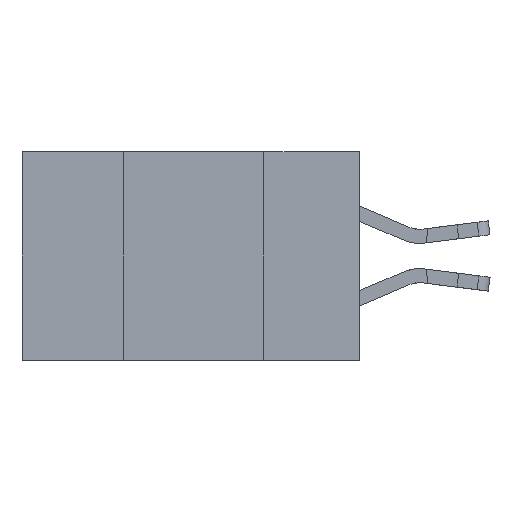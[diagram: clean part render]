
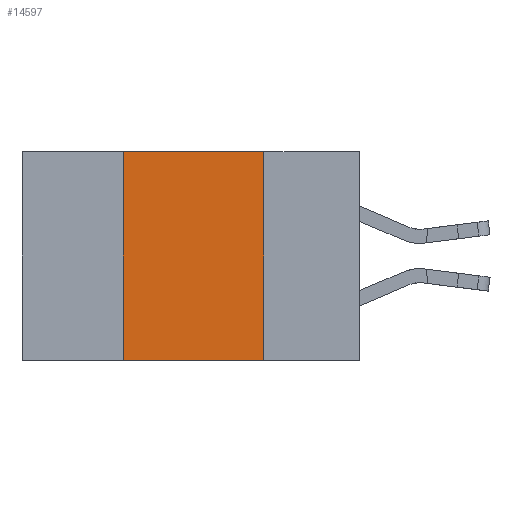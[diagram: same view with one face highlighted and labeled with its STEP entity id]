
A CAD part, left-side view. The second image highlights one B-rep face of the part: STEP entity #14597.
In plain terms, the highlighted planar face has unit normal (-1, 0, 0).
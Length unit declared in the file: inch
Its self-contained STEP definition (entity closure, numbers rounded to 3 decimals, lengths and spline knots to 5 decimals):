
#105 = FACE_OUTER_BOUND ( 'NONE', #21071, .T. ) ;
#202 = ORIENTED_EDGE ( 'NONE', *, *, #13890, .T. ) ;
#730 = DIRECTION ( 'NONE',  ( 0., 0., 1. ) ) ;
#1035 = CARTESIAN_POINT ( 'NONE',  ( 0., 0.42, -0.37 ) ) ;
#1326 = DIRECTION ( 'NONE',  ( 1., 0., 0. ) ) ;
#1566 = DIRECTION ( 'NONE',  ( 0., -1., 0. ) ) ;
#2985 = DIRECTION ( 'NONE',  ( 0., 0., -1. ) ) ;
#4285 = CARTESIAN_POINT ( 'NONE',  ( 0., 0.6, 0. ) ) ;
#6379 = VECTOR ( 'NONE', #1566, 39.37008 ) ;
#7774 = EDGE_CURVE ( 'NONE', #9730, #18237, #19618, .T. ) ;
#7858 = ORIENTED_EDGE ( 'NONE', *, *, #7774, .F. ) ;
#8973 = CARTESIAN_POINT ( 'NONE',  ( 0., 0.17, -0.37 ) ) ;
#9730 = VERTEX_POINT ( 'NONE', #22725 ) ;
#10866 = ORIENTED_EDGE ( 'NONE', *, *, #15050, .F. ) ;
#11631 = VERTEX_POINT ( 'NONE', #8973 ) ;
#12085 = CARTESIAN_POINT ( 'NONE',  ( 0., 0.6, 0. ) ) ;
#13846 = DIRECTION ( 'NONE',  ( 0., 0., -1. ) ) ;
#13890 = EDGE_CURVE ( 'NONE', #20618, #11631, #20948, .T. ) ;
#14597 = ADVANCED_FACE ( 'NONE', ( #105 ), #22437, .F. ) ;
#15050 = EDGE_CURVE ( 'NONE', #20618, #9730, #18485, .T. ) ;
#15930 = AXIS2_PLACEMENT_3D ( 'NONE', #12085, #1326, #13846 ) ;
#17936 = VECTOR ( 'NONE', #730, 39.37008 ) ;
#18013 = VECTOR ( 'NONE', #2985, 39.37008 ) ;
#18189 = CARTESIAN_POINT ( 'NONE',  ( 0., 0.17, 0. ) ) ;
#18237 = VERTEX_POINT ( 'NONE', #18189 ) ;
#18307 = ORIENTED_EDGE ( 'NONE', *, *, #19258, .F. ) ;
#18485 = LINE ( 'NONE', #21829, #17936 ) ;
#18550 = VECTOR ( 'NONE', #20149, 39.37008 ) ;
#18829 = CARTESIAN_POINT ( 'NONE',  ( 0., 0.17, 0. ) ) ;
#19258 = EDGE_CURVE ( 'NONE', #18237, #11631, #22570, .T. ) ;
#19618 = LINE ( 'NONE', #4285, #18550 ) ;
#20149 = DIRECTION ( 'NONE',  ( 0., -1., 0. ) ) ;
#20618 = VERTEX_POINT ( 'NONE', #1035 ) ;
#20948 = LINE ( 'NONE', #22650, #6379 ) ;
#21071 = EDGE_LOOP ( 'NONE', ( #18307, #7858, #10866, #202 ) ) ;
#21829 = CARTESIAN_POINT ( 'NONE',  ( 0., 0.42, 0. ) ) ;
#22437 = PLANE ( 'NONE',  #15930 ) ;
#22570 = LINE ( 'NONE', #18829, #18013 ) ;
#22650 = CARTESIAN_POINT ( 'NONE',  ( 0., 0.6, -0.37 ) ) ;
#22725 = CARTESIAN_POINT ( 'NONE',  ( 0., 0.42, 0. ) ) ;
